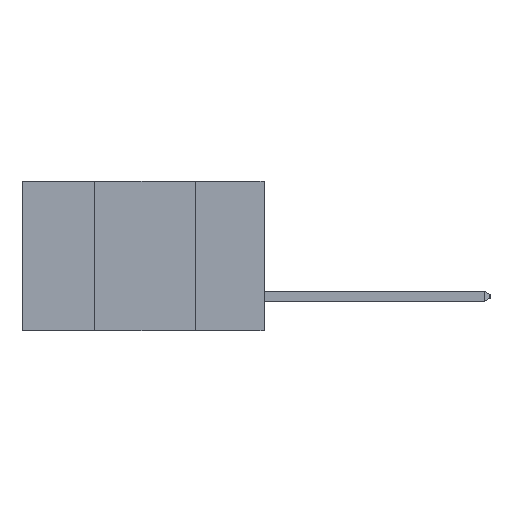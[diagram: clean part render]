
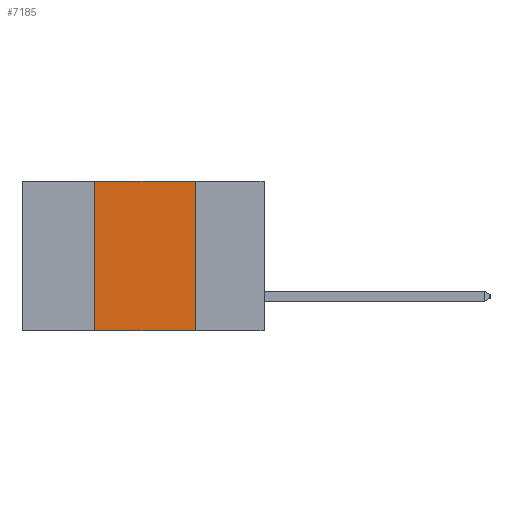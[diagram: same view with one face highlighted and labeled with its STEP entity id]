
A CAD part, left-side view. The second image highlights one B-rep face of the part: STEP entity #7185.
In plain terms, the highlighted planar face has unit normal (-1, 0, 0).
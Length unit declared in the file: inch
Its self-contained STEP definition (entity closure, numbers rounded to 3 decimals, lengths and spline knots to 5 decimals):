
#1069 = DIRECTION ( 'NONE',  ( 1., 0., 0. ) ) ;
#1524 = LINE ( 'NONE', #5678, #13269 ) ;
#2053 = VERTEX_POINT ( 'NONE', #3947 ) ;
#2486 = CARTESIAN_POINT ( 'NONE',  ( 0., 0.42, 0. ) ) ;
#2763 = ORIENTED_EDGE ( 'NONE', *, *, #10690, .F. ) ;
#3234 = VERTEX_POINT ( 'NONE', #11866 ) ;
#3603 = VECTOR ( 'NONE', #14497, 39.37008 ) ;
#3947 = CARTESIAN_POINT ( 'NONE',  ( 0., 0.42, 0. ) ) ;
#4029 = EDGE_CURVE ( 'NONE', #3234, #14132, #1524, .T. ) ;
#4263 = ORIENTED_EDGE ( 'NONE', *, *, #4029, .T. ) ;
#4996 = AXIS2_PLACEMENT_3D ( 'NONE', #12483, #1069, #9196 ) ;
#5537 = CARTESIAN_POINT ( 'NONE',  ( 0., 0.17, 0. ) ) ;
#5678 = CARTESIAN_POINT ( 'NONE',  ( 0., 0.6, -0.37 ) ) ;
#5754 = DIRECTION ( 'NONE',  ( 0., -1., 0. ) ) ;
#5813 = FACE_OUTER_BOUND ( 'NONE', #10304, .T. ) ;
#6213 = LINE ( 'NONE', #2486, #9225 ) ;
#6301 = EDGE_CURVE ( 'NONE', #3234, #2053, #6213, .T. ) ;
#6690 = VECTOR ( 'NONE', #14736, 39.37008 ) ;
#6772 = CARTESIAN_POINT ( 'NONE',  ( 0., 0.17, 0. ) ) ;
#7185 = ADVANCED_FACE ( 'NONE', ( #5813 ), #14643, .F. ) ;
#9196 = DIRECTION ( 'NONE',  ( 0., 0., -1. ) ) ;
#9225 = VECTOR ( 'NONE', #11589, 39.37008 ) ;
#9291 = LINE ( 'NONE', #6772, #3603 ) ;
#9690 = LINE ( 'NONE', #13676, #6690 ) ;
#10304 = EDGE_LOOP ( 'NONE', ( #12321, #2763, #12497, #4263 ) ) ;
#10466 = VERTEX_POINT ( 'NONE', #5537 ) ;
#10690 = EDGE_CURVE ( 'NONE', #2053, #10466, #9690, .T. ) ;
#11557 = EDGE_CURVE ( 'NONE', #10466, #14132, #9291, .T. ) ;
#11589 = DIRECTION ( 'NONE',  ( 0., 0., 1. ) ) ;
#11866 = CARTESIAN_POINT ( 'NONE',  ( 0., 0.42, -0.37 ) ) ;
#11925 = CARTESIAN_POINT ( 'NONE',  ( 0., 0.17, -0.37 ) ) ;
#12321 = ORIENTED_EDGE ( 'NONE', *, *, #11557, .F. ) ;
#12483 = CARTESIAN_POINT ( 'NONE',  ( 0., 0.6, 0. ) ) ;
#12497 = ORIENTED_EDGE ( 'NONE', *, *, #6301, .F. ) ;
#13269 = VECTOR ( 'NONE', #5754, 39.37008 ) ;
#13676 = CARTESIAN_POINT ( 'NONE',  ( 0., 0.6, 0. ) ) ;
#14132 = VERTEX_POINT ( 'NONE', #11925 ) ;
#14497 = DIRECTION ( 'NONE',  ( 0., 0., -1. ) ) ;
#14643 = PLANE ( 'NONE',  #4996 ) ;
#14736 = DIRECTION ( 'NONE',  ( 0., -1., 0. ) ) ;
